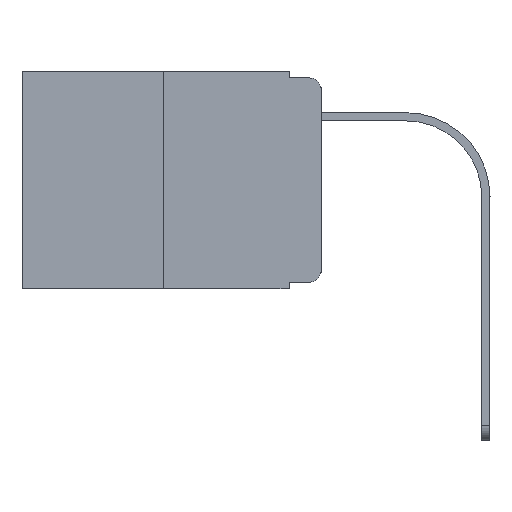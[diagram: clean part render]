
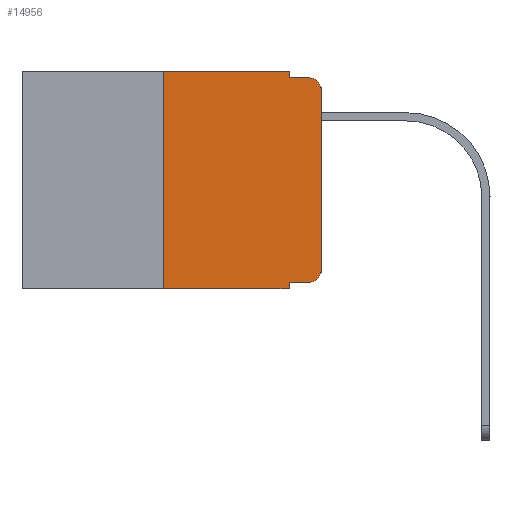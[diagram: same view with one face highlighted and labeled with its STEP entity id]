
A CAD part, left-side view. The second image highlights one B-rep face of the part: STEP entity #14956.
In plain terms, the highlighted planar face has unit normal (-1, 0, 0).
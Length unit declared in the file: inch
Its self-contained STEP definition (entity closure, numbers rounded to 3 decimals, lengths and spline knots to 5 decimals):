
#117 = DIRECTION ( 'NONE',  ( 0., 0., 1. ) ) ;
#927 = CARTESIAN_POINT ( 'NONE',  ( 0., 0.473, -0.343 ) ) ;
#939 = DIRECTION ( 'NONE',  ( 0., -1., 0. ) ) ;
#1007 = CIRCLE ( 'NONE', #17138, 0.02 ) ;
#1063 = DIRECTION ( 'NONE',  ( 1., 0., 0. ) ) ;
#1544 = CARTESIAN_POINT ( 'NONE',  ( 0., 0.25, 0. ) ) ;
#1582 = VECTOR ( 'NONE', #3866, 39.37008 ) ;
#1913 = EDGE_CURVE ( 'NONE', #2568, #16901, #14231, .T. ) ;
#1951 = CARTESIAN_POINT ( 'NONE',  ( 0., 0., 0. ) ) ;
#1999 = VERTEX_POINT ( 'NONE', #17405 ) ;
#2188 = VECTOR ( 'NONE', #12563, 39.37008 ) ;
#2251 = VERTEX_POINT ( 'NONE', #5398 ) ;
#2568 = VERTEX_POINT ( 'NONE', #11623 ) ;
#2614 = CARTESIAN_POINT ( 'NONE',  ( 0., 0.25, -0.343 ) ) ;
#2659 = LINE ( 'NONE', #1544, #7153 ) ;
#2905 = CARTESIAN_POINT ( 'NONE',  ( 0., 0.02, -0.01 ) ) ;
#2942 = EDGE_LOOP ( 'NONE', ( #4656, #13244, #16688, #4456, #18305, #9174, #4354, #10641, #18287, #6547 ) ) ;
#3120 = DIRECTION ( 'NONE',  ( 0., 0., -1. ) ) ;
#3866 = DIRECTION ( 'NONE',  ( 0., 0., -1. ) ) ;
#3902 = CIRCLE ( 'NONE', #8996, 0.02 ) ;
#4065 = CARTESIAN_POINT ( 'NONE',  ( 0., 0.051, -0.343 ) ) ;
#4354 = ORIENTED_EDGE ( 'NONE', *, *, #4673, .T. ) ;
#4401 = CARTESIAN_POINT ( 'NONE',  ( 0., 0.051, -0.01 ) ) ;
#4456 = ORIENTED_EDGE ( 'NONE', *, *, #9575, .F. ) ;
#4515 = DIRECTION ( 'NONE',  ( -1., 0., 0. ) ) ;
#4656 = ORIENTED_EDGE ( 'NONE', *, *, #14392, .T. ) ;
#4673 = EDGE_CURVE ( 'NONE', #6404, #5435, #14973, .T. ) ;
#4837 = LINE ( 'NONE', #1951, #6069 ) ;
#4938 = CARTESIAN_POINT ( 'NONE',  ( 0., 0.02, -0.333 ) ) ;
#5174 = FACE_OUTER_BOUND ( 'NONE', #2942, .T. ) ;
#5178 = CARTESIAN_POINT ( 'NONE',  ( 0., 0.051, 0. ) ) ;
#5367 = EDGE_CURVE ( 'NONE', #6404, #1999, #2659, .T. ) ;
#5398 = CARTESIAN_POINT ( 'NONE',  ( 0., 0.051, -0.333 ) ) ;
#5435 = VERTEX_POINT ( 'NONE', #4065 ) ;
#5518 = CARTESIAN_POINT ( 'NONE',  ( 0., 0.051, -0.333 ) ) ;
#5740 = CARTESIAN_POINT ( 'NONE',  ( 0., 0.051, 0. ) ) ;
#6069 = VECTOR ( 'NONE', #9225, 39.37008 ) ;
#6082 = VECTOR ( 'NONE', #939, 39.37008 ) ;
#6404 = VERTEX_POINT ( 'NONE', #2614 ) ;
#6547 = ORIENTED_EDGE ( 'NONE', *, *, #13561, .T. ) ;
#6847 = CARTESIAN_POINT ( 'NONE',  ( 0., 0.473, 0. ) ) ;
#7153 = VECTOR ( 'NONE', #117, 39.37008 ) ;
#7789 = EDGE_CURVE ( 'NONE', #9823, #16901, #3902, .T. ) ;
#7867 = DIRECTION ( 'NONE',  ( 0., -1., 0. ) ) ;
#8173 = CARTESIAN_POINT ( 'NONE',  ( 0., 0.473, 0. ) ) ;
#8264 = LINE ( 'NONE', #6847, #2188 ) ;
#8736 = VERTEX_POINT ( 'NONE', #13428 ) ;
#8863 = LINE ( 'NONE', #13784, #9947 ) ;
#8996 = AXIS2_PLACEMENT_3D ( 'NONE', #12231, #15219, #10723 ) ;
#9174 = ORIENTED_EDGE ( 'NONE', *, *, #5367, .F. ) ;
#9225 = DIRECTION ( 'NONE',  ( 0., 0., 1. ) ) ;
#9575 = EDGE_CURVE ( 'NONE', #11043, #2568, #11750, .T. ) ;
#9684 = EDGE_CURVE ( 'NONE', #1999, #11043, #8264, .T. ) ;
#9823 = VERTEX_POINT ( 'NONE', #12662 ) ;
#9947 = VECTOR ( 'NONE', #17566, 39.37008 ) ;
#10111 = CARTESIAN_POINT ( 'NONE',  ( 0., 0.02, -0.313 ) ) ;
#10435 = VECTOR ( 'NONE', #15360, 39.37008 ) ;
#10641 = ORIENTED_EDGE ( 'NONE', *, *, #13193, .F. ) ;
#10723 = DIRECTION ( 'NONE',  ( 0., 0., -1. ) ) ;
#11043 = VERTEX_POINT ( 'NONE', #5740 ) ;
#11052 = PLANE ( 'NONE',  #17445 ) ;
#11623 = CARTESIAN_POINT ( 'NONE',  ( 0., 0.051, -0.01 ) ) ;
#11750 = LINE ( 'NONE', #5178, #1582 ) ;
#12135 = VERTEX_POINT ( 'NONE', #4938 ) ;
#12231 = CARTESIAN_POINT ( 'NONE',  ( 0., 0.02, -0.03 ) ) ;
#12563 = DIRECTION ( 'NONE',  ( 0., -1., 0. ) ) ;
#12662 = CARTESIAN_POINT ( 'NONE',  ( 0., 0., -0.03 ) ) ;
#13193 = EDGE_CURVE ( 'NONE', #2251, #5435, #8863, .T. ) ;
#13244 = ORIENTED_EDGE ( 'NONE', *, *, #7789, .T. ) ;
#13428 = CARTESIAN_POINT ( 'NONE',  ( 0., 0., -0.313 ) ) ;
#13561 = EDGE_CURVE ( 'NONE', #12135, #8736, #1007, .T. ) ;
#13616 = DIRECTION ( 'NONE',  ( 0., 0., -1. ) ) ;
#13754 = EDGE_CURVE ( 'NONE', #2251, #12135, #18408, .T. ) ;
#13784 = CARTESIAN_POINT ( 'NONE',  ( 0., 0.051, 0. ) ) ;
#14231 = LINE ( 'NONE', #4401, #10435 ) ;
#14392 = EDGE_CURVE ( 'NONE', #8736, #9823, #4837, .T. ) ;
#14956 = ADVANCED_FACE ( 'NONE', ( #5174 ), #11052, .F. ) ;
#14973 = LINE ( 'NONE', #927, #15758 ) ;
#15219 = DIRECTION ( 'NONE',  ( -1., 0., 0. ) ) ;
#15360 = DIRECTION ( 'NONE',  ( 0., -1., 0. ) ) ;
#15758 = VECTOR ( 'NONE', #7867, 39.37008 ) ;
#16688 = ORIENTED_EDGE ( 'NONE', *, *, #1913, .F. ) ;
#16901 = VERTEX_POINT ( 'NONE', #2905 ) ;
#17138 = AXIS2_PLACEMENT_3D ( 'NONE', #10111, #4515, #3120 ) ;
#17405 = CARTESIAN_POINT ( 'NONE',  ( 0., 0.25, 0. ) ) ;
#17445 = AXIS2_PLACEMENT_3D ( 'NONE', #8173, #1063, #13616 ) ;
#17566 = DIRECTION ( 'NONE',  ( 0., 0., -1. ) ) ;
#18287 = ORIENTED_EDGE ( 'NONE', *, *, #13754, .T. ) ;
#18305 = ORIENTED_EDGE ( 'NONE', *, *, #9684, .F. ) ;
#18408 = LINE ( 'NONE', #5518, #6082 ) ;
